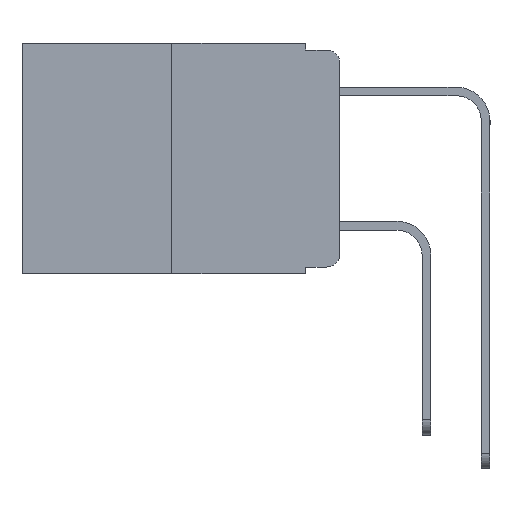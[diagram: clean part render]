
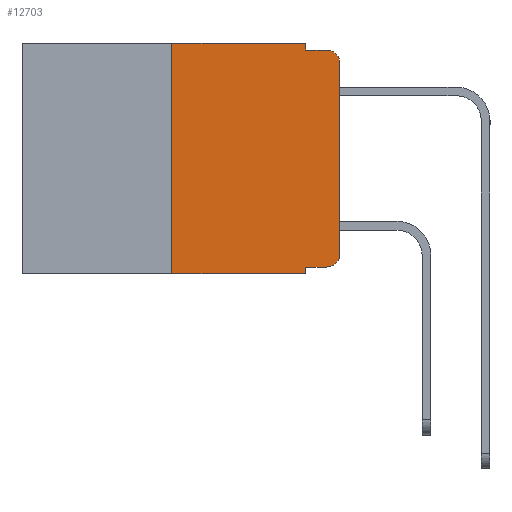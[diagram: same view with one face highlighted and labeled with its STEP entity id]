
A CAD part, left-side view. The second image highlights one B-rep face of the part: STEP entity #12703.
In plain terms, the highlighted planar face has unit normal (-1, 0, 0).
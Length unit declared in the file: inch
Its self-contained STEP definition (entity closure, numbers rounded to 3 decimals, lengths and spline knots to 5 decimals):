
#44 = CARTESIAN_POINT ( 'NONE',  ( 0., 0.051, 0. ) ) ;
#324 = CIRCLE ( 'NONE', #14413, 0.02 ) ;
#644 = EDGE_CURVE ( 'NONE', #11824, #3915, #2988, .T. ) ;
#659 = CARTESIAN_POINT ( 'NONE',  ( 0., 0.051, -0.333 ) ) ;
#811 = CARTESIAN_POINT ( 'NONE',  ( 0., 0.051, 0. ) ) ;
#1291 = VERTEX_POINT ( 'NONE', #6373 ) ;
#1327 = LINE ( 'NONE', #10115, #4734 ) ;
#2218 = VECTOR ( 'NONE', #17025, 39.37008 ) ;
#2416 = VERTEX_POINT ( 'NONE', #44 ) ;
#2750 = EDGE_CURVE ( 'NONE', #16018, #15081, #324, .T. ) ;
#2988 = LINE ( 'NONE', #9989, #16580 ) ;
#3168 = CARTESIAN_POINT ( 'NONE',  ( 0., 0.02, -0.313 ) ) ;
#3915 = VERTEX_POINT ( 'NONE', #10069 ) ;
#4161 = ORIENTED_EDGE ( 'NONE', *, *, #8475, .F. ) ;
#4452 = CARTESIAN_POINT ( 'NONE',  ( 0., 0.473, 0. ) ) ;
#4462 = DIRECTION ( 'NONE',  ( 0., -1., 0. ) ) ;
#4603 = DIRECTION ( 'NONE',  ( 0., 0., -1. ) ) ;
#4648 = EDGE_CURVE ( 'NONE', #2416, #10361, #6919, .T. ) ;
#4734 = VECTOR ( 'NONE', #6231, 39.37008 ) ;
#4901 = CARTESIAN_POINT ( 'NONE',  ( 0., 0., 0. ) ) ;
#4950 = FACE_OUTER_BOUND ( 'NONE', #12013, .T. ) ;
#5193 = EDGE_CURVE ( 'NONE', #1291, #14014, #12195, .T. ) ;
#5221 = ORIENTED_EDGE ( 'NONE', *, *, #10309, .T. ) ;
#5645 = ORIENTED_EDGE ( 'NONE', *, *, #5193, .T. ) ;
#5823 = DIRECTION ( 'NONE',  ( 1., 0., 0. ) ) ;
#5871 = LINE ( 'NONE', #16062, #12388 ) ;
#5943 = LINE ( 'NONE', #8797, #15910 ) ;
#6231 = DIRECTION ( 'NONE',  ( 0., -1., 0. ) ) ;
#6373 = CARTESIAN_POINT ( 'NONE',  ( 0., 0., -0.03 ) ) ;
#6521 = VECTOR ( 'NONE', #11717, 39.37008 ) ;
#6883 = CARTESIAN_POINT ( 'NONE',  ( 0., 0.02, -0.333 ) ) ;
#6900 = ORIENTED_EDGE ( 'NONE', *, *, #2750, .T. ) ;
#6919 = LINE ( 'NONE', #811, #6521 ) ;
#7348 = DIRECTION ( 'NONE',  ( 0., 0., 1. ) ) ;
#7454 = CARTESIAN_POINT ( 'NONE',  ( 0., 0., -0.313 ) ) ;
#7467 = VERTEX_POINT ( 'NONE', #659 ) ;
#7511 = ORIENTED_EDGE ( 'NONE', *, *, #9839, .T. ) ;
#7573 = CARTESIAN_POINT ( 'NONE',  ( 0., 0.25, -0.343 ) ) ;
#7952 = DIRECTION ( 'NONE',  ( -1., 0., 0. ) ) ;
#8035 = CARTESIAN_POINT ( 'NONE',  ( 0., 0.051, 0. ) ) ;
#8174 = ORIENTED_EDGE ( 'NONE', *, *, #14459, .F. ) ;
#8255 = EDGE_CURVE ( 'NONE', #7467, #11765, #16703, .T. ) ;
#8410 = ORIENTED_EDGE ( 'NONE', *, *, #8255, .F. ) ;
#8439 = CARTESIAN_POINT ( 'NONE',  ( 0., 0.051, -0.01 ) ) ;
#8475 = EDGE_CURVE ( 'NONE', #10361, #14014, #9244, .T. ) ;
#8738 = CARTESIAN_POINT ( 'NONE',  ( 0., 0.051, -0.343 ) ) ;
#8797 = CARTESIAN_POINT ( 'NONE',  ( 0., 0.473, 0. ) ) ;
#9244 = LINE ( 'NONE', #13641, #12682 ) ;
#9839 = EDGE_CURVE ( 'NONE', #15081, #1291, #13634, .T. ) ;
#9989 = CARTESIAN_POINT ( 'NONE',  ( 0., 0.25, 0. ) ) ;
#10069 = CARTESIAN_POINT ( 'NONE',  ( 0., 0.25, 0. ) ) ;
#10115 = CARTESIAN_POINT ( 'NONE',  ( 0., 0.473, -0.343 ) ) ;
#10309 = EDGE_CURVE ( 'NONE', #7467, #16018, #5871, .T. ) ;
#10361 = VERTEX_POINT ( 'NONE', #8439 ) ;
#11717 = DIRECTION ( 'NONE',  ( 0., 0., -1. ) ) ;
#11765 = VERTEX_POINT ( 'NONE', #8738 ) ;
#11824 = VERTEX_POINT ( 'NONE', #7573 ) ;
#12013 = EDGE_LOOP ( 'NONE', ( #7511, #5645, #4161, #12606, #8174, #16635, #13452, #8410, #5221, #6900 ) ) ;
#12195 = CIRCLE ( 'NONE', #14670, 0.02 ) ;
#12388 = VECTOR ( 'NONE', #17293, 39.37008 ) ;
#12448 = DIRECTION ( 'NONE',  ( -1., 0., 0. ) ) ;
#12606 = ORIENTED_EDGE ( 'NONE', *, *, #4648, .F. ) ;
#12682 = VECTOR ( 'NONE', #4462, 39.37008 ) ;
#12703 = ADVANCED_FACE ( 'NONE', ( #4950 ), #16154, .F. ) ;
#12890 = EDGE_CURVE ( 'NONE', #11824, #11765, #1327, .T. ) ;
#13218 = VECTOR ( 'NONE', #7348, 39.37008 ) ;
#13452 = ORIENTED_EDGE ( 'NONE', *, *, #12890, .T. ) ;
#13634 = LINE ( 'NONE', #4901, #13218 ) ;
#13641 = CARTESIAN_POINT ( 'NONE',  ( 0., 0.051, -0.01 ) ) ;
#13696 = CARTESIAN_POINT ( 'NONE',  ( 0., 0.02, -0.01 ) ) ;
#14014 = VERTEX_POINT ( 'NONE', #13696 ) ;
#14413 = AXIS2_PLACEMENT_3D ( 'NONE', #3168, #12448, #4603 ) ;
#14459 = EDGE_CURVE ( 'NONE', #3915, #2416, #5943, .T. ) ;
#14670 = AXIS2_PLACEMENT_3D ( 'NONE', #15720, #7952, #16961 ) ;
#14936 = DIRECTION ( 'NONE',  ( 0., 0., -1. ) ) ;
#15081 = VERTEX_POINT ( 'NONE', #7454 ) ;
#15319 = DIRECTION ( 'NONE',  ( 0., -1., 0. ) ) ;
#15720 = CARTESIAN_POINT ( 'NONE',  ( 0., 0.02, -0.03 ) ) ;
#15910 = VECTOR ( 'NONE', #15319, 39.37008 ) ;
#16018 = VERTEX_POINT ( 'NONE', #6883 ) ;
#16062 = CARTESIAN_POINT ( 'NONE',  ( 0., 0.051, -0.333 ) ) ;
#16154 = PLANE ( 'NONE',  #16660 ) ;
#16580 = VECTOR ( 'NONE', #16836, 39.37008 ) ;
#16635 = ORIENTED_EDGE ( 'NONE', *, *, #644, .F. ) ;
#16660 = AXIS2_PLACEMENT_3D ( 'NONE', #4452, #5823, #14936 ) ;
#16703 = LINE ( 'NONE', #8035, #2218 ) ;
#16836 = DIRECTION ( 'NONE',  ( 0., 0., 1. ) ) ;
#16961 = DIRECTION ( 'NONE',  ( 0., 0., -1. ) ) ;
#17025 = DIRECTION ( 'NONE',  ( 0., 0., -1. ) ) ;
#17293 = DIRECTION ( 'NONE',  ( 0., -1., 0. ) ) ;
